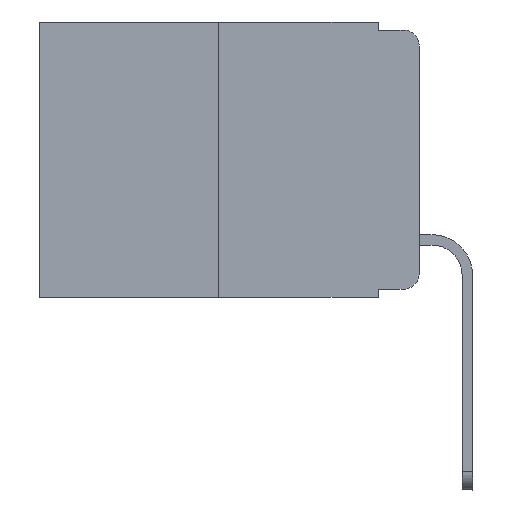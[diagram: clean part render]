
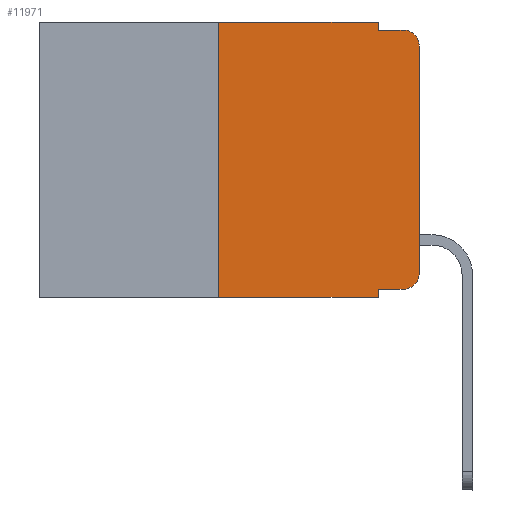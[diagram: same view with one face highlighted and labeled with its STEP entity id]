
A CAD part, left-side view. The second image highlights one B-rep face of the part: STEP entity #11971.
In plain terms, the highlighted planar face has unit normal (-1, 0, 0).
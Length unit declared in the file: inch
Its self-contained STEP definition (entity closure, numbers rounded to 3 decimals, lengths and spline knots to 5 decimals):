
#267 = ORIENTED_EDGE ( 'NONE', *, *, #3065, .T. ) ;
#364 = CARTESIAN_POINT ( 'NONE',  ( 0., 0.051, 0. ) ) ;
#572 = ORIENTED_EDGE ( 'NONE', *, *, #9474, .F. ) ;
#959 = CIRCLE ( 'NONE', #4997, 0.02 ) ;
#992 = VECTOR ( 'NONE', #6433, 39.37008 ) ;
#1036 = DIRECTION ( 'NONE',  ( 1., 0., 0. ) ) ;
#1572 = VERTEX_POINT ( 'NONE', #10230 ) ;
#1640 = ORIENTED_EDGE ( 'NONE', *, *, #8091, .T. ) ;
#1780 = ORIENTED_EDGE ( 'NONE', *, *, #9982, .F. ) ;
#2391 = VERTEX_POINT ( 'NONE', #5543 ) ;
#2528 = EDGE_CURVE ( 'NONE', #8451, #7235, #7719, .T. ) ;
#2555 = DIRECTION ( 'NONE',  ( -1., 0., 0. ) ) ;
#2650 = ORIENTED_EDGE ( 'NONE', *, *, #3565, .F. ) ;
#2685 = VECTOR ( 'NONE', #5209, 39.37008 ) ;
#2702 = VERTEX_POINT ( 'NONE', #5020 ) ;
#2732 = ORIENTED_EDGE ( 'NONE', *, *, #4902, .T. ) ;
#2838 = DIRECTION ( 'NONE',  ( 0., -1., 0. ) ) ;
#3014 = CARTESIAN_POINT ( 'NONE',  ( 0., 0., -0.313 ) ) ;
#3065 = EDGE_CURVE ( 'NONE', #1572, #2702, #959, .T. ) ;
#3554 = LINE ( 'NONE', #10908, #10417 ) ;
#3565 = EDGE_CURVE ( 'NONE', #8451, #5693, #12121, .T. ) ;
#3678 = CARTESIAN_POINT ( 'NONE',  ( 0., 0.02, -0.313 ) ) ;
#3865 = FACE_OUTER_BOUND ( 'NONE', #10138, .T. ) ;
#3918 = DIRECTION ( 'NONE',  ( -1., 0., 0. ) ) ;
#3970 = DIRECTION ( 'NONE',  ( 0., 0., 1. ) ) ;
#4397 = CARTESIAN_POINT ( 'NONE',  ( 0., 0.051, -0.01 ) ) ;
#4733 = DIRECTION ( 'NONE',  ( 0., 0., 1. ) ) ;
#4902 = EDGE_CURVE ( 'NONE', #7235, #11656, #7056, .T. ) ;
#4997 = AXIS2_PLACEMENT_3D ( 'NONE', #8968, #3918, #6904 ) ;
#5020 = CARTESIAN_POINT ( 'NONE',  ( 0., 0.02, -0.01 ) ) ;
#5124 = LINE ( 'NONE', #9102, #12562 ) ;
#5148 = ORIENTED_EDGE ( 'NONE', *, *, #10791, .F. ) ;
#5209 = DIRECTION ( 'NONE',  ( 0., -1., 0. ) ) ;
#5369 = CARTESIAN_POINT ( 'NONE',  ( 0., 0.051, 0. ) ) ;
#5471 = VECTOR ( 'NONE', #3970, 39.37008 ) ;
#5543 = CARTESIAN_POINT ( 'NONE',  ( 0., 0.25, 0. ) ) ;
#5693 = VERTEX_POINT ( 'NONE', #11670 ) ;
#5813 = DIRECTION ( 'NONE',  ( 0., 0., -1. ) ) ;
#6116 = CARTESIAN_POINT ( 'NONE',  ( 0., 0.051, 0. ) ) ;
#6271 = ORIENTED_EDGE ( 'NONE', *, *, #2528, .T. ) ;
#6302 = LINE ( 'NONE', #5369, #992 ) ;
#6419 = DIRECTION ( 'NONE',  ( 0., 0., -1. ) ) ;
#6433 = DIRECTION ( 'NONE',  ( 0., 0., -1. ) ) ;
#6618 = VERTEX_POINT ( 'NONE', #364 ) ;
#6675 = DIRECTION ( 'NONE',  ( 0., -1., 0. ) ) ;
#6768 = CARTESIAN_POINT ( 'NONE',  ( 0., 0.25, 0. ) ) ;
#6837 = AXIS2_PLACEMENT_3D ( 'NONE', #3678, #2555, #6419 ) ;
#6857 = CARTESIAN_POINT ( 'NONE',  ( 0., 0.051, -0.333 ) ) ;
#6904 = DIRECTION ( 'NONE',  ( 0., 0., -1. ) ) ;
#7054 = CARTESIAN_POINT ( 'NONE',  ( 0., 0.473, 0. ) ) ;
#7056 = CIRCLE ( 'NONE', #6837, 0.02 ) ;
#7192 = EDGE_CURVE ( 'NONE', #9677, #2391, #9819, .T. ) ;
#7235 = VERTEX_POINT ( 'NONE', #7892 ) ;
#7420 = CARTESIAN_POINT ( 'NONE',  ( 0., 0.25, -0.343 ) ) ;
#7596 = DIRECTION ( 'NONE',  ( 0., -1., 0. ) ) ;
#7719 = LINE ( 'NONE', #6857, #9925 ) ;
#7892 = CARTESIAN_POINT ( 'NONE',  ( 0., 0.02, -0.333 ) ) ;
#8091 = EDGE_CURVE ( 'NONE', #9677, #5693, #3554, .T. ) ;
#8118 = PLANE ( 'NONE',  #10525 ) ;
#8218 = CARTESIAN_POINT ( 'NONE',  ( 0., 0.051, -0.333 ) ) ;
#8241 = CARTESIAN_POINT ( 'NONE',  ( 0., 0.051, -0.01 ) ) ;
#8451 = VERTEX_POINT ( 'NONE', #8218 ) ;
#8968 = CARTESIAN_POINT ( 'NONE',  ( 0., 0.02, -0.03 ) ) ;
#9102 = CARTESIAN_POINT ( 'NONE',  ( 0., 0.473, 0. ) ) ;
#9194 = VERTEX_POINT ( 'NONE', #4397 ) ;
#9474 = EDGE_CURVE ( 'NONE', #2391, #6618, #5124, .T. ) ;
#9677 = VERTEX_POINT ( 'NONE', #7420 ) ;
#9819 = LINE ( 'NONE', #6768, #11241 ) ;
#9925 = VECTOR ( 'NONE', #6675, 39.37008 ) ;
#9982 = EDGE_CURVE ( 'NONE', #6618, #9194, #6302, .T. ) ;
#10081 = ORIENTED_EDGE ( 'NONE', *, *, #7192, .F. ) ;
#10138 = EDGE_LOOP ( 'NONE', ( #10547, #267, #5148, #1780, #572, #10081, #1640, #2650, #6271, #2732 ) ) ;
#10142 = DIRECTION ( 'NONE',  ( 0., 0., -1. ) ) ;
#10194 = CARTESIAN_POINT ( 'NONE',  ( 0., 0., 0. ) ) ;
#10230 = CARTESIAN_POINT ( 'NONE',  ( 0., 0., -0.03 ) ) ;
#10417 = VECTOR ( 'NONE', #7596, 39.37008 ) ;
#10525 = AXIS2_PLACEMENT_3D ( 'NONE', #7054, #1036, #5813 ) ;
#10547 = ORIENTED_EDGE ( 'NONE', *, *, #11171, .T. ) ;
#10791 = EDGE_CURVE ( 'NONE', #9194, #2702, #11530, .T. ) ;
#10908 = CARTESIAN_POINT ( 'NONE',  ( 0., 0.473, -0.343 ) ) ;
#11171 = EDGE_CURVE ( 'NONE', #11656, #1572, #12119, .T. ) ;
#11241 = VECTOR ( 'NONE', #4733, 39.37008 ) ;
#11530 = LINE ( 'NONE', #8241, #2685 ) ;
#11605 = VECTOR ( 'NONE', #10142, 39.37008 ) ;
#11656 = VERTEX_POINT ( 'NONE', #3014 ) ;
#11670 = CARTESIAN_POINT ( 'NONE',  ( 0., 0.051, -0.343 ) ) ;
#11971 = ADVANCED_FACE ( 'NONE', ( #3865 ), #8118, .F. ) ;
#12119 = LINE ( 'NONE', #10194, #5471 ) ;
#12121 = LINE ( 'NONE', #6116, #11605 ) ;
#12562 = VECTOR ( 'NONE', #2838, 39.37008 ) ;
